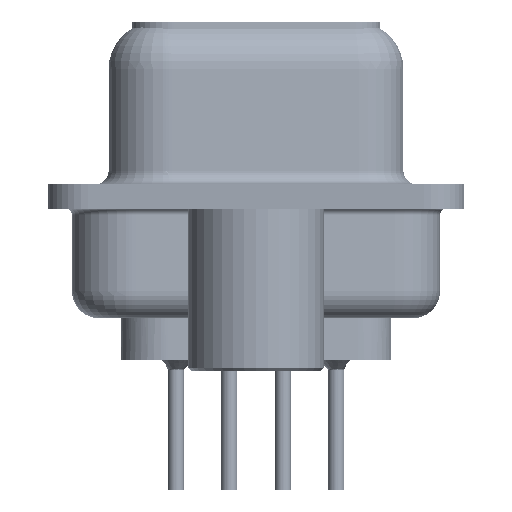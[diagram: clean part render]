
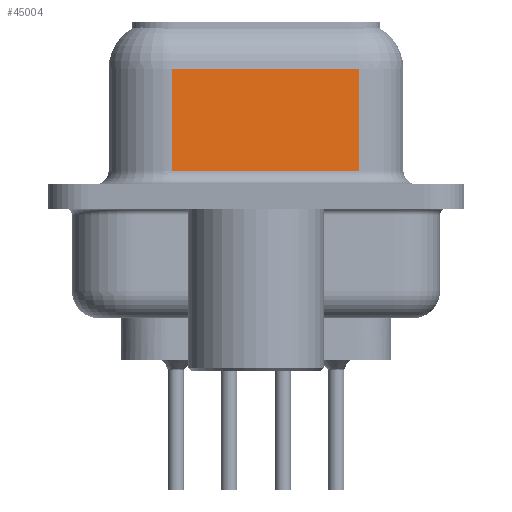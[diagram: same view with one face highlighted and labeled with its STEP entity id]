
A CAD part, left-side view. The second image highlights one B-rep face of the part: STEP entity #45004.
In plain terms, the highlighted planar face has unit normal (-0.985, -0.174, 0).
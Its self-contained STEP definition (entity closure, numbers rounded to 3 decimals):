
#465 = ORIENTED_EDGE ( 'NONE', *, *, #39838, .T. ) ;
#4850 = AXIS2_PLACEMENT_3D ( 'NONE', #15784, #47478, #14627 ) ;
#8245 = VECTOR ( 'NONE', #53224, 1000. ) ;
#8341 = ORIENTED_EDGE ( 'NONE', *, *, #51745, .F. ) ;
#10611 = DIRECTION ( 'NONE',  ( 0., 0., -1. ) ) ;
#13014 = VERTEX_POINT ( 'NONE', #33785 ) ;
#14627 = DIRECTION ( 'NONE',  ( -0.174, 0.985, 0. ) ) ;
#15007 = LINE ( 'NONE', #19451, #23768 ) ;
#15784 = CARTESIAN_POINT ( 'NONE',  ( 5.697, -3.797, 6.45 ) ) ;
#15855 = CARTESIAN_POINT ( 'NONE',  ( 5.697, -3.797, 0.95 ) ) ;
#17698 = EDGE_CURVE ( 'NONE', #13014, #50084, #41974, .T. ) ;
#18220 = VECTOR ( 'NONE', #54127, 1000. ) ;
#19451 = CARTESIAN_POINT ( 'NONE',  ( 5.697, -3.797, 6.45 ) ) ;
#22960 = EDGE_CURVE ( 'NONE', #50084, #38992, #45715, .T. ) ;
#23768 = VECTOR ( 'NONE', #10611, 1000. ) ;
#23890 = DIRECTION ( 'NONE',  ( 0.174, -0.985, 0. ) ) ;
#29414 = PLANE ( 'NONE',  #4850 ) ;
#33785 = CARTESIAN_POINT ( 'NONE',  ( 5.697, -3.797, 4.7 ) ) ;
#35137 = CARTESIAN_POINT ( 'NONE',  ( 4.48, 3.103, 6.45 ) ) ;
#35234 = CARTESIAN_POINT ( 'NONE',  ( 4.48, 3.103, 0.95 ) ) ;
#36059 = CARTESIAN_POINT ( 'NONE',  ( 5.697, -3.797, 4.7 ) ) ;
#37149 = ORIENTED_EDGE ( 'NONE', *, *, #22960, .T. ) ;
#37297 = VERTEX_POINT ( 'NONE', #55987 ) ;
#38892 = EDGE_LOOP ( 'NONE', ( #8341, #39748, #37149, #465 ) ) ;
#38992 = VERTEX_POINT ( 'NONE', #35234 ) ;
#39748 = ORIENTED_EDGE ( 'NONE', *, *, #17698, .T. ) ;
#39838 = EDGE_CURVE ( 'NONE', #38992, #37297, #55572, .T. ) ;
#41974 = LINE ( 'NONE', #36059, #18220 ) ;
#45004 = ADVANCED_FACE ( 'NONE', ( #55787 ), #29414, .F. ) ;
#45715 = LINE ( 'NONE', #35137, #8245 ) ;
#47478 = DIRECTION ( 'NONE',  ( 0.985, 0.174, 0. ) ) ;
#50084 = VERTEX_POINT ( 'NONE', #57317 ) ;
#51745 = EDGE_CURVE ( 'NONE', #13014, #37297, #15007, .T. ) ;
#53224 = DIRECTION ( 'NONE',  ( 0., 0., -1. ) ) ;
#54127 = DIRECTION ( 'NONE',  ( -0.174, 0.985, 0. ) ) ;
#55572 = LINE ( 'NONE', #15855, #56976 ) ;
#55787 = FACE_OUTER_BOUND ( 'NONE', #38892, .T. ) ;
#55987 = CARTESIAN_POINT ( 'NONE',  ( 5.697, -3.797, 0.95 ) ) ;
#56976 = VECTOR ( 'NONE', #23890, 1000. ) ;
#57317 = CARTESIAN_POINT ( 'NONE',  ( 4.48, 3.103, 4.7 ) ) ;
